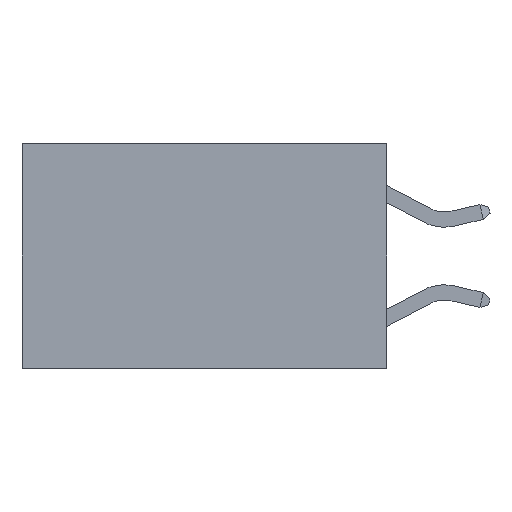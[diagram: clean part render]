
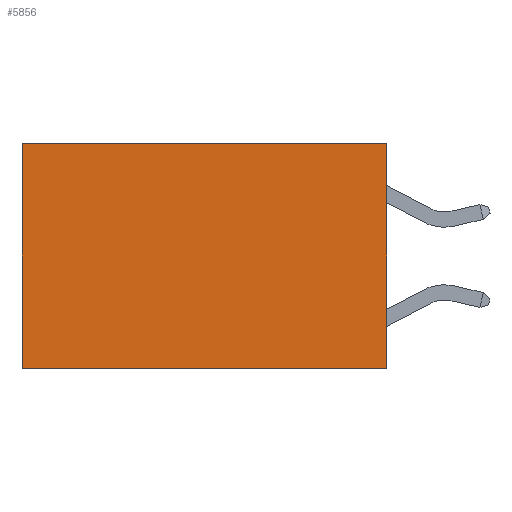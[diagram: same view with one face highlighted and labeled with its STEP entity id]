
A CAD part, left-side view. The second image highlights one B-rep face of the part: STEP entity #5856.
In plain terms, the highlighted planar face has unit normal (-1, 0, 0).
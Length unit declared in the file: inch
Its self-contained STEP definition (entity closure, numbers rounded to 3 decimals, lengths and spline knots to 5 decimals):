
#747 = ORIENTED_EDGE ( 'NONE', *, *, #8122, .T. ) ;
#953 = CARTESIAN_POINT ( 'NONE',  ( 0.2625, 0.6, 0. ) ) ;
#1366 = CARTESIAN_POINT ( 'NONE',  ( 0.2625, 0., -0.37 ) ) ;
#1507 = ORIENTED_EDGE ( 'NONE', *, *, #4081, .F. ) ;
#1941 = EDGE_CURVE ( 'NONE', #2023, #10882, #4672, .T. ) ;
#2023 = VERTEX_POINT ( 'NONE', #3976 ) ;
#2047 = LINE ( 'NONE', #9317, #10859 ) ;
#2134 = VECTOR ( 'NONE', #7267, 39.37008 ) ;
#3462 = VERTEX_POINT ( 'NONE', #9352 ) ;
#3907 = DIRECTION ( 'NONE',  ( 0., 1., 0. ) ) ;
#3976 = CARTESIAN_POINT ( 'NONE',  ( 0.2625, 0.6, 0. ) ) ;
#4081 = EDGE_CURVE ( 'NONE', #10085, #10882, #7117, .T. ) ;
#4232 = DIRECTION ( 'NONE',  ( 1., 0., 0. ) ) ;
#4325 = CARTESIAN_POINT ( 'NONE',  ( 0.2625, 0.6, -0.37 ) ) ;
#4514 = ORIENTED_EDGE ( 'NONE', *, *, #1941, .T. ) ;
#4576 = VECTOR ( 'NONE', #3907, 39.37008 ) ;
#4672 = LINE ( 'NONE', #953, #2134 ) ;
#4961 = EDGE_CURVE ( 'NONE', #3462, #10085, #2047, .T. ) ;
#5281 = DIRECTION ( 'NONE',  ( 0., 0., -1. ) ) ;
#5856 = ADVANCED_FACE ( 'NONE', ( #10095 ), #9231, .F. ) ;
#5941 = ORIENTED_EDGE ( 'NONE', *, *, #4961, .F. ) ;
#5971 = CARTESIAN_POINT ( 'NONE',  ( 0.2625, 0., -0.37 ) ) ;
#6502 = CARTESIAN_POINT ( 'NONE',  ( 0.2625, 0., 0. ) ) ;
#6588 = LINE ( 'NONE', #6502, #4576 ) ;
#7117 = LINE ( 'NONE', #1366, #9507 ) ;
#7267 = DIRECTION ( 'NONE',  ( 0., 0., -1. ) ) ;
#8122 = EDGE_CURVE ( 'NONE', #3462, #2023, #6588, .T. ) ;
#8362 = DIRECTION ( 'NONE',  ( 0., 1., 0. ) ) ;
#8394 = CARTESIAN_POINT ( 'NONE',  ( 0.2625, 0., 0. ) ) ;
#9231 = PLANE ( 'NONE',  #9642 ) ;
#9317 = CARTESIAN_POINT ( 'NONE',  ( 0.2625, 0., 0. ) ) ;
#9352 = CARTESIAN_POINT ( 'NONE',  ( 0.2625, 0., 0. ) ) ;
#9507 = VECTOR ( 'NONE', #8362, 39.37008 ) ;
#9642 = AXIS2_PLACEMENT_3D ( 'NONE', #8394, #4232, #10016 ) ;
#10016 = DIRECTION ( 'NONE',  ( 0., 0., -1. ) ) ;
#10085 = VERTEX_POINT ( 'NONE', #5971 ) ;
#10095 = FACE_OUTER_BOUND ( 'NONE', #10245, .T. ) ;
#10245 = EDGE_LOOP ( 'NONE', ( #4514, #1507, #5941, #747 ) ) ;
#10859 = VECTOR ( 'NONE', #5281, 39.37008 ) ;
#10882 = VERTEX_POINT ( 'NONE', #4325 ) ;
